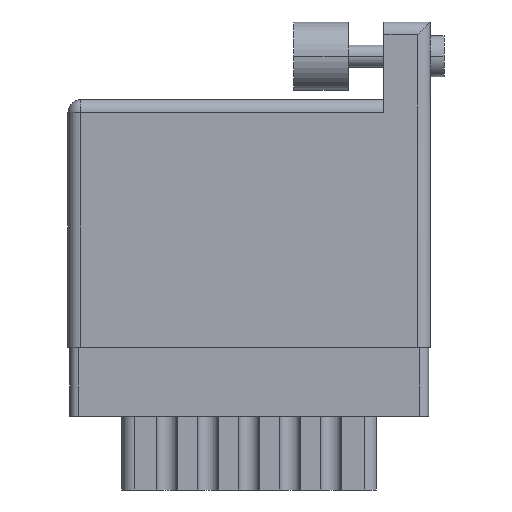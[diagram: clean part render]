
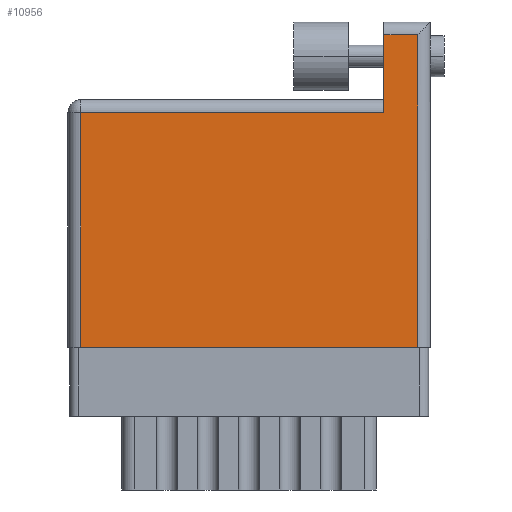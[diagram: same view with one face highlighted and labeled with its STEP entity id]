
A CAD part, front view. The second image highlights one B-rep face of the part: STEP entity #10956.
In plain terms, the highlighted face is planar.
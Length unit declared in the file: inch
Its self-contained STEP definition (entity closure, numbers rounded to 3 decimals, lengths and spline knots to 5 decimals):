
#298 = CARTESIAN_POINT ( 'NONE',  ( 1.278, 1.143, 0. ) ) ;
#391 = CARTESIAN_POINT ( 'NONE',  ( 1.155, 1.143, 0. ) ) ;
#403 = EDGE_CURVE ( 'NONE', #11199, #13650, #10019, .T. ) ;
#549 = CARTESIAN_POINT ( 'NONE',  ( 0.047, 0., 0. ) ) ;
#1067 = CARTESIAN_POINT ( 'NONE',  ( 0., 0.906, 0. ) ) ;
#1155 = FACE_OUTER_BOUND ( 'NONE', #6175, .T. ) ;
#1747 = ORIENTED_EDGE ( 'NONE', *, *, #16333, .T. ) ;
#2214 = VERTEX_POINT ( 'NONE', #298 ) ;
#2236 = ORIENTED_EDGE ( 'NONE', *, *, #6150, .T. ) ;
#2279 = VECTOR ( 'NONE', #10809, 39.37008 ) ;
#2464 = DIRECTION ( 'NONE',  ( 0., 1., 0. ) ) ;
#2592 = LINE ( 'NONE', #16755, #13824 ) ;
#2810 = CARTESIAN_POINT ( 'NONE',  ( 1.278, 0., 0. ) ) ;
#3881 = DIRECTION ( 'NONE',  ( -1., 0., 0. ) ) ;
#4345 = EDGE_CURVE ( 'NONE', #10896, #10570, #7439, .T. ) ;
#4832 = LINE ( 'NONE', #5199, #2279 ) ;
#5199 = CARTESIAN_POINT ( 'NONE',  ( 0., 0., 0. ) ) ;
#5576 = VECTOR ( 'NONE', #10384, 39.37008 ) ;
#5849 = EDGE_CURVE ( 'NONE', #13650, #11114, #4832, .T. ) ;
#6150 = EDGE_CURVE ( 'NONE', #2214, #10896, #7386, .T. ) ;
#6175 = EDGE_LOOP ( 'NONE', ( #8114, #15185, #2236, #12292, #1747, #17724 ) ) ;
#6586 = DIRECTION ( 'NONE',  ( -1., 0., 0. ) ) ;
#6904 = AXIS2_PLACEMENT_3D ( 'NONE', #1067, #10905, #6586 ) ;
#7133 = LINE ( 'NONE', #9898, #12407 ) ;
#7386 = LINE ( 'NONE', #391, #8446 ) ;
#7439 = LINE ( 'NONE', #16359, #13398 ) ;
#7591 = CARTESIAN_POINT ( 'NONE',  ( 0.047, 0.859, 0. ) ) ;
#7801 = DIRECTION ( 'NONE',  ( 0., -1., 0. ) ) ;
#7875 = PLANE ( 'NONE',  #6904 ) ;
#8114 = ORIENTED_EDGE ( 'NONE', *, *, #5849, .T. ) ;
#8446 = VECTOR ( 'NONE', #11629, 39.37008 ) ;
#9898 = CARTESIAN_POINT ( 'NONE',  ( 1.278, 1.19, 0. ) ) ;
#10019 = LINE ( 'NONE', #549, #5576 ) ;
#10384 = DIRECTION ( 'NONE',  ( 0., -1., 0. ) ) ;
#10570 = VERTEX_POINT ( 'NONE', #15251 ) ;
#10762 = CARTESIAN_POINT ( 'NONE',  ( 0.047, 0., 0. ) ) ;
#10809 = DIRECTION ( 'NONE',  ( 1., 0., 0. ) ) ;
#10896 = VERTEX_POINT ( 'NONE', #13582 ) ;
#10905 = DIRECTION ( 'NONE',  ( 0., 0., -1. ) ) ;
#10956 = ADVANCED_FACE ( 'NONE', ( #1155 ), #7875, .F. ) ;
#11114 = VERTEX_POINT ( 'NONE', #2810 ) ;
#11199 = VERTEX_POINT ( 'NONE', #7591 ) ;
#11629 = DIRECTION ( 'NONE',  ( -1., 0., 0. ) ) ;
#12292 = ORIENTED_EDGE ( 'NONE', *, *, #4345, .T. ) ;
#12300 = EDGE_CURVE ( 'NONE', #11114, #2214, #7133, .T. ) ;
#12407 = VECTOR ( 'NONE', #2464, 39.37008 ) ;
#13398 = VECTOR ( 'NONE', #7801, 39.37008 ) ;
#13582 = CARTESIAN_POINT ( 'NONE',  ( 1.155, 1.143, 0. ) ) ;
#13650 = VERTEX_POINT ( 'NONE', #10762 ) ;
#13824 = VECTOR ( 'NONE', #3881, 39.37008 ) ;
#15185 = ORIENTED_EDGE ( 'NONE', *, *, #12300, .T. ) ;
#15251 = CARTESIAN_POINT ( 'NONE',  ( 1.155, 0.859, 0. ) ) ;
#16333 = EDGE_CURVE ( 'NONE', #10570, #11199, #2592, .T. ) ;
#16359 = CARTESIAN_POINT ( 'NONE',  ( 1.155, 1.19, 0. ) ) ;
#16755 = CARTESIAN_POINT ( 'NONE',  ( 0., 0.859, 0. ) ) ;
#17724 = ORIENTED_EDGE ( 'NONE', *, *, #403, .T. ) ;
